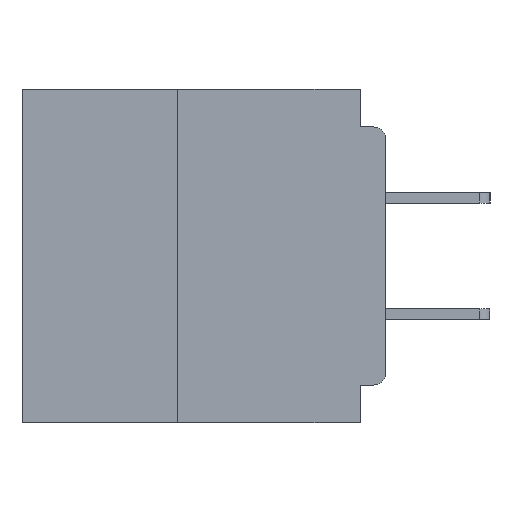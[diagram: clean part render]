
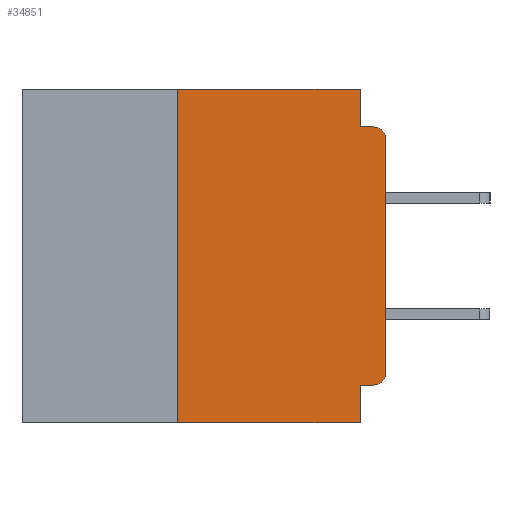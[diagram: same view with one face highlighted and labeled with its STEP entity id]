
A CAD part, left-side view. The second image highlights one B-rep face of the part: STEP entity #34851.
In plain terms, the highlighted planar face has unit normal (-1, 0, 0).
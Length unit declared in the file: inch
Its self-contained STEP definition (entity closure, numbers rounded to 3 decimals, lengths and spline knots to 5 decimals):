
#685 = CARTESIAN_POINT ( 'NONE',  ( 0., 0.437, 0. ) ) ;
#883 = VECTOR ( 'NONE', #12221, 39.37008 ) ;
#902 = ORIENTED_EDGE ( 'NONE', *, *, #28247, .F. ) ;
#1909 = DIRECTION ( 'NONE',  ( 0., -1., 0. ) ) ;
#4053 = CARTESIAN_POINT ( 'NONE',  ( 0., 0.031, -0.355 ) ) ;
#5235 = CARTESIAN_POINT ( 'NONE',  ( 0., 0.015, -0.355 ) ) ;
#6268 = ORIENTED_EDGE ( 'NONE', *, *, #51804, .F. ) ;
#6682 = CARTESIAN_POINT ( 'NONE',  ( 0., 0.031, 0. ) ) ;
#7129 = ORIENTED_EDGE ( 'NONE', *, *, #23070, .T. ) ;
#7869 = CARTESIAN_POINT ( 'NONE',  ( 0., 0., -0.045 ) ) ;
#8370 = VERTEX_POINT ( 'NONE', #48162 ) ;
#8594 = LINE ( 'NONE', #18407, #51012 ) ;
#8832 = LINE ( 'NONE', #9051, #30704 ) ;
#9051 = CARTESIAN_POINT ( 'NONE',  ( 0., 0.437, 0. ) ) ;
#9053 = ORIENTED_EDGE ( 'NONE', *, *, #29515, .T. ) ;
#9084 = DIRECTION ( 'NONE',  ( 1., 0., 0. ) ) ;
#10037 = CARTESIAN_POINT ( 'NONE',  ( 0., 0.25, 0. ) ) ;
#10096 = VERTEX_POINT ( 'NONE', #23177 ) ;
#10147 = CIRCLE ( 'NONE', #40413, 0.015 ) ;
#11026 = VECTOR ( 'NONE', #32447, 39.37008 ) ;
#11807 = CARTESIAN_POINT ( 'NONE',  ( 0., 0., 0. ) ) ;
#12221 = DIRECTION ( 'NONE',  ( 0., -1., 0. ) ) ;
#13419 = CARTESIAN_POINT ( 'NONE',  ( 0., 0.015, -0.34 ) ) ;
#13546 = CARTESIAN_POINT ( 'NONE',  ( 0., 0., -0.06 ) ) ;
#14440 = EDGE_CURVE ( 'NONE', #46671, #8370, #8832, .T. ) ;
#14999 = DIRECTION ( 'NONE',  ( 0., 0., -1. ) ) ;
#15534 = CIRCLE ( 'NONE', #42842, 0.015 ) ;
#15704 = LINE ( 'NONE', #6682, #37532 ) ;
#15858 = VECTOR ( 'NONE', #43262, 39.37008 ) ;
#16534 = LINE ( 'NONE', #29680, #35731 ) ;
#17542 = DIRECTION ( 'NONE',  ( 0., 0., -1. ) ) ;
#17767 = CARTESIAN_POINT ( 'NONE',  ( 0., 0., -0.34 ) ) ;
#18001 = CARTESIAN_POINT ( 'NONE',  ( 0., 0.015, -0.06 ) ) ;
#18407 = CARTESIAN_POINT ( 'NONE',  ( 0., 0.437, -0.4 ) ) ;
#18756 = ORIENTED_EDGE ( 'NONE', *, *, #20564, .F. ) ;
#20564 = EDGE_CURVE ( 'NONE', #38657, #10096, #33830, .T. ) ;
#20576 = VERTEX_POINT ( 'NONE', #4053 ) ;
#21743 = ORIENTED_EDGE ( 'NONE', *, *, #47270, .F. ) ;
#21947 = LINE ( 'NONE', #11807, #11026 ) ;
#22107 = DIRECTION ( 'NONE',  ( 0., 0., -1. ) ) ;
#22190 = DIRECTION ( 'NONE',  ( 0., 0., 1. ) ) ;
#22786 = CARTESIAN_POINT ( 'NONE',  ( 0., 0.031, -0.4 ) ) ;
#23070 = EDGE_CURVE ( 'NONE', #35524, #10096, #10147, .T. ) ;
#23177 = CARTESIAN_POINT ( 'NONE',  ( 0., 0.015, -0.045 ) ) ;
#25155 = ORIENTED_EDGE ( 'NONE', *, *, #42035, .T. ) ;
#25384 = AXIS2_PLACEMENT_3D ( 'NONE', #685, #9084, #37833 ) ;
#28247 = EDGE_CURVE ( 'NONE', #20576, #31192, #48604, .T. ) ;
#29515 = EDGE_CURVE ( 'NONE', #49322, #31192, #8594, .T. ) ;
#29642 = LINE ( 'NONE', #50932, #40537 ) ;
#29680 = CARTESIAN_POINT ( 'NONE',  ( 0., 0., -0.355 ) ) ;
#30704 = VECTOR ( 'NONE', #37807, 39.37008 ) ;
#31192 = VERTEX_POINT ( 'NONE', #51672 ) ;
#32204 = CARTESIAN_POINT ( 'NONE',  ( 0., 0.25, -0.4 ) ) ;
#32447 = DIRECTION ( 'NONE',  ( 0., 0., 1. ) ) ;
#32545 = CARTESIAN_POINT ( 'NONE',  ( 0., 0.031, -0.045 ) ) ;
#32770 = ORIENTED_EDGE ( 'NONE', *, *, #41828, .T. ) ;
#33707 = PLANE ( 'NONE',  #25384 ) ;
#33830 = LINE ( 'NONE', #7869, #883 ) ;
#34851 = ADVANCED_FACE ( 'NONE', ( #42204 ), #33707, .F. ) ;
#35524 = VERTEX_POINT ( 'NONE', #13546 ) ;
#35731 = VECTOR ( 'NONE', #42003, 39.37008 ) ;
#37532 = VECTOR ( 'NONE', #14999, 39.37008 ) ;
#37807 = DIRECTION ( 'NONE',  ( 0., -1., 0. ) ) ;
#37833 = DIRECTION ( 'NONE',  ( 0., 0., -1. ) ) ;
#38657 = VERTEX_POINT ( 'NONE', #32545 ) ;
#40413 = AXIS2_PLACEMENT_3D ( 'NONE', #18001, #46721, #22107 ) ;
#40537 = VECTOR ( 'NONE', #22190, 39.37008 ) ;
#41828 = EDGE_CURVE ( 'NONE', #50321, #35524, #21947, .T. ) ;
#42003 = DIRECTION ( 'NONE',  ( 0., 1., 0. ) ) ;
#42035 = EDGE_CURVE ( 'NONE', #48920, #50321, #15534, .T. ) ;
#42076 = DIRECTION ( 'NONE',  ( -1., 0., 0. ) ) ;
#42204 = FACE_OUTER_BOUND ( 'NONE', #45766, .T. ) ;
#42842 = AXIS2_PLACEMENT_3D ( 'NONE', #13419, #42076, #17542 ) ;
#43262 = DIRECTION ( 'NONE',  ( 0., 0., -1. ) ) ;
#44786 = ORIENTED_EDGE ( 'NONE', *, *, #14440, .F. ) ;
#45766 = EDGE_LOOP ( 'NONE', ( #32770, #7129, #18756, #6268, #44786, #21743, #9053, #902, #52487, #25155 ) ) ;
#46671 = VERTEX_POINT ( 'NONE', #10037 ) ;
#46721 = DIRECTION ( 'NONE',  ( -1., 0., 0. ) ) ;
#47270 = EDGE_CURVE ( 'NONE', #49322, #46671, #29642, .T. ) ;
#48162 = CARTESIAN_POINT ( 'NONE',  ( 0., 0.031, 0. ) ) ;
#48604 = LINE ( 'NONE', #22786, #15858 ) ;
#48920 = VERTEX_POINT ( 'NONE', #5235 ) ;
#49322 = VERTEX_POINT ( 'NONE', #32204 ) ;
#50321 = VERTEX_POINT ( 'NONE', #17767 ) ;
#50379 = EDGE_CURVE ( 'NONE', #48920, #20576, #16534, .T. ) ;
#50932 = CARTESIAN_POINT ( 'NONE',  ( 0., 0.25, -0.4 ) ) ;
#51012 = VECTOR ( 'NONE', #1909, 39.37008 ) ;
#51672 = CARTESIAN_POINT ( 'NONE',  ( 0., 0.031, -0.4 ) ) ;
#51804 = EDGE_CURVE ( 'NONE', #8370, #38657, #15704, .T. ) ;
#52487 = ORIENTED_EDGE ( 'NONE', *, *, #50379, .F. ) ;
